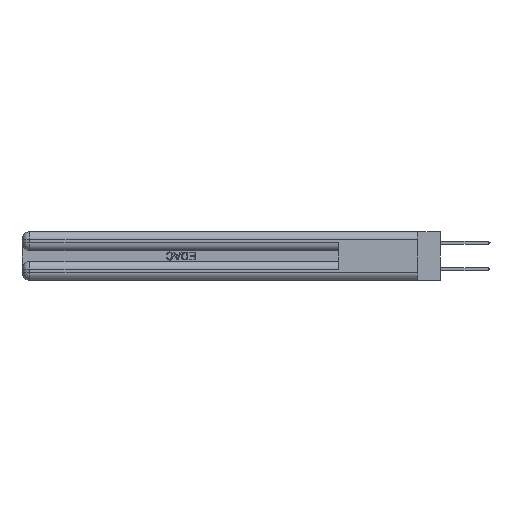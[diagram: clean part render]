
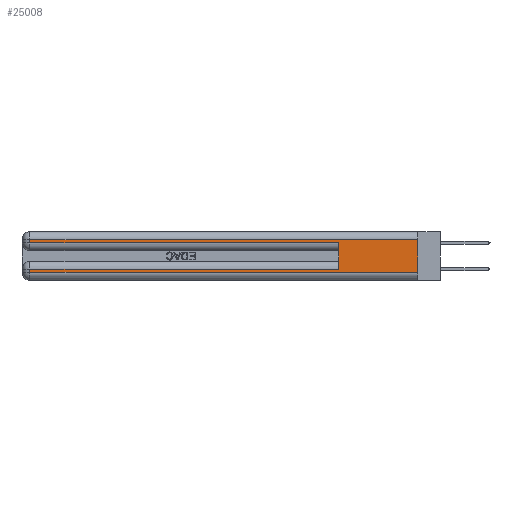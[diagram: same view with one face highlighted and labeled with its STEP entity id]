
A CAD part, left-side view. The second image highlights one B-rep face of the part: STEP entity #25008.
In plain terms, the highlighted planar face has unit normal (-1, 0, 0).
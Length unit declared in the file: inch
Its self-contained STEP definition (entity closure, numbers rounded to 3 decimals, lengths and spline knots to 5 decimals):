
#106 = ORIENTED_EDGE ( 'NONE', *, *, #40561, .T. ) ;
#747 = VECTOR ( 'NONE', #46999, 39.37008 ) ;
#1381 = CARTESIAN_POINT ( 'NONE',  ( 0., 0., 0.085 ) ) ;
#2070 = VERTEX_POINT ( 'NONE', #41200 ) ;
#2092 = FACE_OUTER_BOUND ( 'NONE', #6462, .T. ) ;
#3198 = CARTESIAN_POINT ( 'NONE',  ( 0., 0.6, 0.285 ) ) ;
#3307 = EDGE_CURVE ( 'NONE', #10872, #26042, #29632, .T. ) ;
#3969 = EDGE_CURVE ( 'NONE', #8508, #10872, #31894, .T. ) ;
#3988 = ORIENTED_EDGE ( 'NONE', *, *, #19127, .T. ) ;
#6022 = DIRECTION ( 'NONE',  ( 0., 1., 0. ) ) ;
#6462 = EDGE_LOOP ( 'NONE', ( #40590, #12342, #13066, #12384, #34718, #3988, #106, #41459 ) ) ;
#8508 = VERTEX_POINT ( 'NONE', #32424 ) ;
#9062 = CARTESIAN_POINT ( 'NONE',  ( 0., 0., 0.31 ) ) ;
#9818 = EDGE_CURVE ( 'NONE', #25407, #8508, #31638, .T. ) ;
#10593 = VERTEX_POINT ( 'NONE', #32481 ) ;
#10681 = LINE ( 'NONE', #1381, #747 ) ;
#10872 = VERTEX_POINT ( 'NONE', #13495 ) ;
#11247 = DIRECTION ( 'NONE',  ( 0., 0., -1. ) ) ;
#11276 = LINE ( 'NONE', #14726, #20545 ) ;
#12051 = VECTOR ( 'NONE', #16610, 39.37008 ) ;
#12342 = ORIENTED_EDGE ( 'NONE', *, *, #9818, .T. ) ;
#12384 = ORIENTED_EDGE ( 'NONE', *, *, #3307, .T. ) ;
#12461 = CARTESIAN_POINT ( 'NONE',  ( 0., 0., 0.285 ) ) ;
#13066 = ORIENTED_EDGE ( 'NONE', *, *, #3969, .T. ) ;
#13495 = CARTESIAN_POINT ( 'NONE',  ( 0., 2.94, 0.285 ) ) ;
#13696 = CARTESIAN_POINT ( 'NONE',  ( 0., 2.94, 0.37 ) ) ;
#14480 = VERTEX_POINT ( 'NONE', #33975 ) ;
#14613 = CARTESIAN_POINT ( 'NONE',  ( 0., 0., 0.37 ) ) ;
#14726 = CARTESIAN_POINT ( 'NONE',  ( 0., 0., 0.06 ) ) ;
#15035 = LINE ( 'NONE', #46680, #42933 ) ;
#15645 = AXIS2_PLACEMENT_3D ( 'NONE', #18316, #44299, #22070 ) ;
#16359 = LINE ( 'NONE', #25997, #16979 ) ;
#16610 = DIRECTION ( 'NONE',  ( 0., 0., -1. ) ) ;
#16979 = VECTOR ( 'NONE', #11247, 39.37008 ) ;
#18209 = EDGE_CURVE ( 'NONE', #25407, #10593, #46226, .T. ) ;
#18316 = CARTESIAN_POINT ( 'NONE',  ( 0., 0., 0.37 ) ) ;
#19127 = EDGE_CURVE ( 'NONE', #2070, #23108, #10681, .T. ) ;
#20545 = VECTOR ( 'NONE', #21720, 39.37008 ) ;
#21012 = DIRECTION ( 'NONE',  ( 0., 0., 1. ) ) ;
#21720 = DIRECTION ( 'NONE',  ( 0., -1., 0. ) ) ;
#21903 = PLANE ( 'NONE',  #15645 ) ;
#22070 = DIRECTION ( 'NONE',  ( 0., 0., -1. ) ) ;
#23108 = VERTEX_POINT ( 'NONE', #48040 ) ;
#23453 = VECTOR ( 'NONE', #6022, 39.37008 ) ;
#23655 = DIRECTION ( 'NONE',  ( 0., -1., 0. ) ) ;
#25008 = ADVANCED_FACE ( 'NONE', ( #2092 ), #21903, .F. ) ;
#25407 = VERTEX_POINT ( 'NONE', #9062 ) ;
#25788 = DIRECTION ( 'NONE',  ( 0., 0., -1. ) ) ;
#25997 = CARTESIAN_POINT ( 'NONE',  ( 0., 2.94, 0.37 ) ) ;
#26042 = VERTEX_POINT ( 'NONE', #3198 ) ;
#27255 = VECTOR ( 'NONE', #23655, 39.37008 ) ;
#28099 = CARTESIAN_POINT ( 'NONE',  ( 0., 0., 0.31 ) ) ;
#28384 = EDGE_CURVE ( 'NONE', #2070, #26042, #15035, .T. ) ;
#29632 = LINE ( 'NONE', #12461, #27255 ) ;
#31638 = LINE ( 'NONE', #28099, #23453 ) ;
#31776 = EDGE_CURVE ( 'NONE', #14480, #10593, #11276, .T. ) ;
#31894 = LINE ( 'NONE', #13696, #12051 ) ;
#32424 = CARTESIAN_POINT ( 'NONE',  ( 0., 2.94, 0.31 ) ) ;
#32481 = CARTESIAN_POINT ( 'NONE',  ( 0., 0., 0.06 ) ) ;
#33975 = CARTESIAN_POINT ( 'NONE',  ( 0., 2.94, 0.06 ) ) ;
#34718 = ORIENTED_EDGE ( 'NONE', *, *, #28384, .F. ) ;
#40561 = EDGE_CURVE ( 'NONE', #23108, #14480, #16359, .T. ) ;
#40590 = ORIENTED_EDGE ( 'NONE', *, *, #18209, .F. ) ;
#41200 = CARTESIAN_POINT ( 'NONE',  ( 0., 0.6, 0.085 ) ) ;
#41459 = ORIENTED_EDGE ( 'NONE', *, *, #31776, .T. ) ;
#42933 = VECTOR ( 'NONE', #21012, 39.37008 ) ;
#44299 = DIRECTION ( 'NONE',  ( 1., 0., 0. ) ) ;
#45042 = VECTOR ( 'NONE', #25788, 39.37008 ) ;
#46226 = LINE ( 'NONE', #14613, #45042 ) ;
#46680 = CARTESIAN_POINT ( 'NONE',  ( 0., 0.6, 0.145 ) ) ;
#46999 = DIRECTION ( 'NONE',  ( 0., 1., 0. ) ) ;
#48040 = CARTESIAN_POINT ( 'NONE',  ( 0., 2.94, 0.085 ) ) ;
